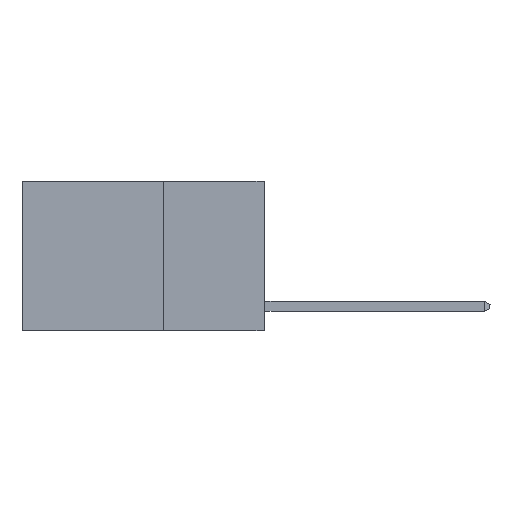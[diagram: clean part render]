
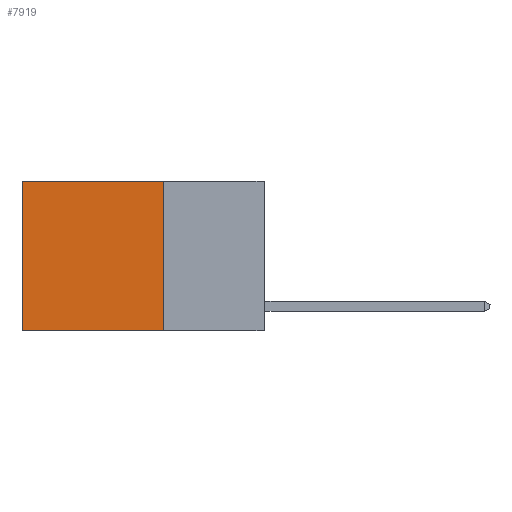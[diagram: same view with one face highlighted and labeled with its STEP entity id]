
A CAD part, left-side view. The second image highlights one B-rep face of the part: STEP entity #7919.
In plain terms, the highlighted planar face has unit normal (-1, 0, 0).
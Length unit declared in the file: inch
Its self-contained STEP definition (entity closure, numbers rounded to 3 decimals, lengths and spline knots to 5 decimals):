
#304 = ORIENTED_EDGE ( 'NONE', *, *, #2348, .F. ) ;
#513 = DIRECTION ( 'NONE',  ( 0., 1., 0. ) ) ;
#994 = DIRECTION ( 'NONE',  ( 0., 0., -1. ) ) ;
#1784 = PLANE ( 'NONE',  #9606 ) ;
#1834 = EDGE_LOOP ( 'NONE', ( #4375, #4138, #304, #9259 ) ) ;
#2348 = EDGE_CURVE ( 'NONE', #3352, #8101, #4707, .T. ) ;
#2390 = VECTOR ( 'NONE', #5350, 39.37008 ) ;
#3352 = VERTEX_POINT ( 'NONE', #4142 ) ;
#3788 = CARTESIAN_POINT ( 'NONE',  ( 0.2625, 0.6, -0.37 ) ) ;
#4138 = ORIENTED_EDGE ( 'NONE', *, *, #10182, .F. ) ;
#4142 = CARTESIAN_POINT ( 'NONE',  ( 0.2625, 0.25, 0. ) ) ;
#4375 = ORIENTED_EDGE ( 'NONE', *, *, #4908, .T. ) ;
#4687 = CARTESIAN_POINT ( 'NONE',  ( 0.2625, 0.25, -0.37 ) ) ;
#4702 = VECTOR ( 'NONE', #513, 39.37008 ) ;
#4707 = LINE ( 'NONE', #8098, #9332 ) ;
#4908 = EDGE_CURVE ( 'NONE', #12603, #12278, #12285, .T. ) ;
#5350 = DIRECTION ( 'NONE',  ( 0., 0., -1. ) ) ;
#6238 = LINE ( 'NONE', #8369, #11290 ) ;
#6346 = CARTESIAN_POINT ( 'NONE',  ( 0.2625, 0.25, -0.37 ) ) ;
#6568 = EDGE_CURVE ( 'NONE', #3352, #12603, #6238, .T. ) ;
#6933 = FACE_OUTER_BOUND ( 'NONE', #1834, .T. ) ;
#7871 = CARTESIAN_POINT ( 'NONE',  ( 0.2625, 0.6, 0. ) ) ;
#7919 = ADVANCED_FACE ( 'NONE', ( #6933 ), #1784, .F. ) ;
#7927 = CARTESIAN_POINT ( 'NONE',  ( 0.2625, 0.25, 0. ) ) ;
#8098 = CARTESIAN_POINT ( 'NONE',  ( 0.2625, 0.25, 0. ) ) ;
#8101 = VERTEX_POINT ( 'NONE', #4687 ) ;
#8369 = CARTESIAN_POINT ( 'NONE',  ( 0.2625, 0.25, 0. ) ) ;
#9259 = ORIENTED_EDGE ( 'NONE', *, *, #6568, .T. ) ;
#9332 = VECTOR ( 'NONE', #994, 39.37008 ) ;
#9606 = AXIS2_PLACEMENT_3D ( 'NONE', #7927, #13937, #13794 ) ;
#9660 = DIRECTION ( 'NONE',  ( 0., 1., 0. ) ) ;
#10182 = EDGE_CURVE ( 'NONE', #8101, #12278, #15334, .T. ) ;
#11290 = VECTOR ( 'NONE', #9660, 39.37008 ) ;
#12040 = CARTESIAN_POINT ( 'NONE',  ( 0.2625, 0.6, 0. ) ) ;
#12278 = VERTEX_POINT ( 'NONE', #3788 ) ;
#12285 = LINE ( 'NONE', #7871, #2390 ) ;
#12603 = VERTEX_POINT ( 'NONE', #12040 ) ;
#13794 = DIRECTION ( 'NONE',  ( 0., 0., -1. ) ) ;
#13937 = DIRECTION ( 'NONE',  ( 1., 0., 0. ) ) ;
#15334 = LINE ( 'NONE', #6346, #4702 ) ;
